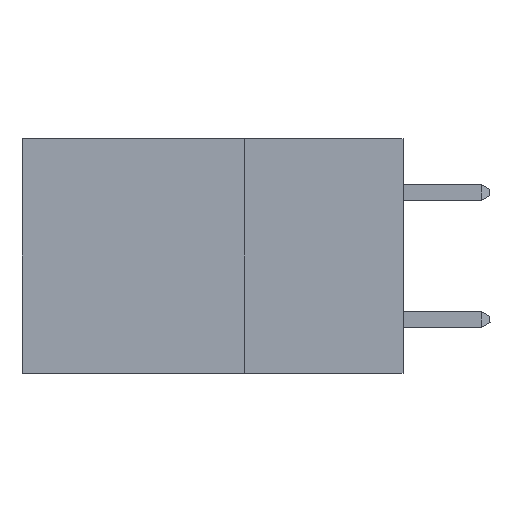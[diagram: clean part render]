
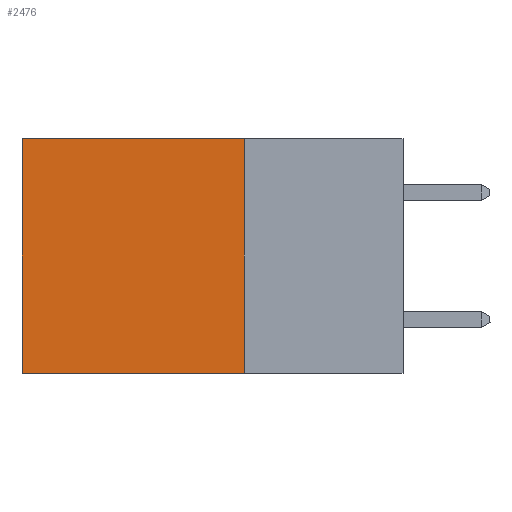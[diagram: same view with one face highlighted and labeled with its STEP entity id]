
A CAD part, left-side view. The second image highlights one B-rep face of the part: STEP entity #2476.
In plain terms, the highlighted planar face has unit normal (-1, 0, 0).
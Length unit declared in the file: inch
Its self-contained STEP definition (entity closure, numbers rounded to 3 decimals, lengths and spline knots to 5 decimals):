
#39 = DIRECTION ( 'NONE',  ( 0., 1., 0. ) ) ;
#80 = CARTESIAN_POINT ( 'NONE',  ( 0.2875, 0.25, -0.37 ) ) ;
#239 = LINE ( 'NONE', #4901, #10259 ) ;
#391 = ORIENTED_EDGE ( 'NONE', *, *, #554, .F. ) ;
#497 = ORIENTED_EDGE ( 'NONE', *, *, #3134, .T. ) ;
#554 = EDGE_CURVE ( 'NONE', #1123, #1677, #4112, .T. ) ;
#625 = CARTESIAN_POINT ( 'NONE',  ( 0.2875, 0.6, 0. ) ) ;
#724 = EDGE_LOOP ( 'NONE', ( #11833, #391, #1105, #497 ) ) ;
#749 = CARTESIAN_POINT ( 'NONE',  ( 0.2875, 0.6, 0. ) ) ;
#1105 = ORIENTED_EDGE ( 'NONE', *, *, #3236, .F. ) ;
#1123 = VERTEX_POINT ( 'NONE', #4073 ) ;
#1328 = DIRECTION ( 'NONE',  ( 0., 0., -1. ) ) ;
#1677 = VERTEX_POINT ( 'NONE', #6109 ) ;
#1695 = EDGE_CURVE ( 'NONE', #2150, #1677, #10731, .T. ) ;
#2150 = VERTEX_POINT ( 'NONE', #749 ) ;
#2476 = ADVANCED_FACE ( 'NONE', ( #11461 ), #5985, .F. ) ;
#2521 = DIRECTION ( 'NONE',  ( 0., 0., -1. ) ) ;
#3134 = EDGE_CURVE ( 'NONE', #3828, #2150, #4636, .T. ) ;
#3236 = EDGE_CURVE ( 'NONE', #3828, #1123, #239, .T. ) ;
#3828 = VERTEX_POINT ( 'NONE', #9480 ) ;
#4073 = CARTESIAN_POINT ( 'NONE',  ( 0.2875, 0.25, -0.37 ) ) ;
#4112 = LINE ( 'NONE', #80, #4837 ) ;
#4636 = LINE ( 'NONE', #9433, #5519 ) ;
#4837 = VECTOR ( 'NONE', #10403, 39.37008 ) ;
#4901 = CARTESIAN_POINT ( 'NONE',  ( 0.2875, 0.25, 0. ) ) ;
#4903 = DIRECTION ( 'NONE',  ( 0., 0., -1. ) ) ;
#4944 = CARTESIAN_POINT ( 'NONE',  ( 0.2875, 0.25, 0. ) ) ;
#5519 = VECTOR ( 'NONE', #39, 39.37008 ) ;
#5985 = PLANE ( 'NONE',  #10127 ) ;
#6109 = CARTESIAN_POINT ( 'NONE',  ( 0.2875, 0.6, -0.37 ) ) ;
#8384 = VECTOR ( 'NONE', #2521, 39.37008 ) ;
#9433 = CARTESIAN_POINT ( 'NONE',  ( 0.2875, 0.25, 0. ) ) ;
#9480 = CARTESIAN_POINT ( 'NONE',  ( 0.2875, 0.25, 0. ) ) ;
#9590 = DIRECTION ( 'NONE',  ( 1., 0., 0. ) ) ;
#10127 = AXIS2_PLACEMENT_3D ( 'NONE', #4944, #9590, #4903 ) ;
#10259 = VECTOR ( 'NONE', #1328, 39.37008 ) ;
#10403 = DIRECTION ( 'NONE',  ( 0., 1., 0. ) ) ;
#10731 = LINE ( 'NONE', #625, #8384 ) ;
#11461 = FACE_OUTER_BOUND ( 'NONE', #724, .T. ) ;
#11833 = ORIENTED_EDGE ( 'NONE', *, *, #1695, .T. ) ;
